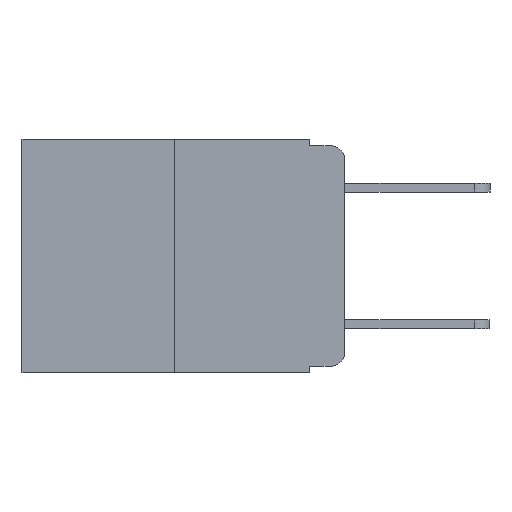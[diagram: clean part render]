
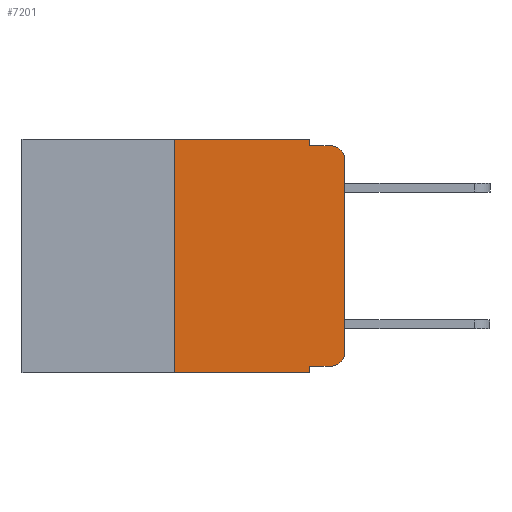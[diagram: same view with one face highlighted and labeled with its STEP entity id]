
A CAD part, left-side view. The second image highlights one B-rep face of the part: STEP entity #7201.
In plain terms, the highlighted planar face has unit normal (-1, 0, 0).
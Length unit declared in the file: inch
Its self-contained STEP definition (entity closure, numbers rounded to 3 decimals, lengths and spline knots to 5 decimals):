
#104 = VERTEX_POINT ( 'NONE', #10284 ) ;
#169 = CARTESIAN_POINT ( 'NONE',  ( 0., 0.051, 0. ) ) ;
#177 = VERTEX_POINT ( 'NONE', #1009 ) ;
#323 = VERTEX_POINT ( 'NONE', #8674 ) ;
#616 = VERTEX_POINT ( 'NONE', #6913 ) ;
#637 = ORIENTED_EDGE ( 'NONE', *, *, #11054, .F. ) ;
#781 = VECTOR ( 'NONE', #5788, 39.37008 ) ;
#1009 = CARTESIAN_POINT ( 'NONE',  ( 0., 0.02, -0.333 ) ) ;
#1039 = VERTEX_POINT ( 'NONE', #5582 ) ;
#1251 = ORIENTED_EDGE ( 'NONE', *, *, #3674, .T. ) ;
#1295 = VERTEX_POINT ( 'NONE', #3208 ) ;
#1386 = DIRECTION ( 'NONE',  ( -1., 0., 0. ) ) ;
#1568 = DIRECTION ( 'NONE',  ( 0., 0., -1. ) ) ;
#1674 = VECTOR ( 'NONE', #9213, 39.37008 ) ;
#1779 = VECTOR ( 'NONE', #10039, 39.37008 ) ;
#1827 = CARTESIAN_POINT ( 'NONE',  ( 0., 0.473, -0.343 ) ) ;
#2004 = LINE ( 'NONE', #1827, #8441 ) ;
#2006 = VERTEX_POINT ( 'NONE', #4079 ) ;
#2091 = ORIENTED_EDGE ( 'NONE', *, *, #7746, .F. ) ;
#2125 = EDGE_CURVE ( 'NONE', #323, #6568, #8767, .T. ) ;
#2162 = DIRECTION ( 'NONE',  ( -1., 0., 0. ) ) ;
#2323 = ORIENTED_EDGE ( 'NONE', *, *, #6759, .F. ) ;
#2906 = LINE ( 'NONE', #7291, #7264 ) ;
#3208 = CARTESIAN_POINT ( 'NONE',  ( 0., 0.25, 0. ) ) ;
#3257 = CIRCLE ( 'NONE', #7239, 0.02 ) ;
#3265 = CARTESIAN_POINT ( 'NONE',  ( 0., 0.051, -0.01 ) ) ;
#3390 = CARTESIAN_POINT ( 'NONE',  ( 0., 0.051, 0. ) ) ;
#3674 = EDGE_CURVE ( 'NONE', #177, #323, #3257, .T. ) ;
#3682 = ORIENTED_EDGE ( 'NONE', *, *, #8267, .F. ) ;
#3972 = VERTEX_POINT ( 'NONE', #10206 ) ;
#4079 = CARTESIAN_POINT ( 'NONE',  ( 0., 0.051, -0.01 ) ) ;
#4178 = PLANE ( 'NONE',  #7007 ) ;
#4637 = LINE ( 'NONE', #9237, #6681 ) ;
#4669 = VECTOR ( 'NONE', #5437, 39.37008 ) ;
#4691 = ORIENTED_EDGE ( 'NONE', *, *, #11189, .F. ) ;
#4791 = VERTEX_POINT ( 'NONE', #3390 ) ;
#4934 = LINE ( 'NONE', #11251, #4669 ) ;
#5046 = DIRECTION ( 'NONE',  ( 1., 0., 0. ) ) ;
#5053 = AXIS2_PLACEMENT_3D ( 'NONE', #6808, #1386, #7648 ) ;
#5229 = FACE_OUTER_BOUND ( 'NONE', #6292, .T. ) ;
#5437 = DIRECTION ( 'NONE',  ( 0., 0., 1. ) ) ;
#5490 = ORIENTED_EDGE ( 'NONE', *, *, #2125, .T. ) ;
#5582 = CARTESIAN_POINT ( 'NONE',  ( 0., 0.051, -0.343 ) ) ;
#5788 = DIRECTION ( 'NONE',  ( 0., 0., -1. ) ) ;
#5792 = ORIENTED_EDGE ( 'NONE', *, *, #6597, .T. ) ;
#5906 = DIRECTION ( 'NONE',  ( 0., -1., 0. ) ) ;
#5909 = EDGE_CURVE ( 'NONE', #104, #1039, #2004, .T. ) ;
#6289 = DIRECTION ( 'NONE',  ( 0., -1., 0. ) ) ;
#6292 = EDGE_LOOP ( 'NONE', ( #5490, #8907, #2323, #3682, #637, #2091, #10070, #4691, #5792, #1251 ) ) ;
#6568 = VERTEX_POINT ( 'NONE', #8056 ) ;
#6597 = EDGE_CURVE ( 'NONE', #616, #177, #2906, .T. ) ;
#6681 = VECTOR ( 'NONE', #5906, 39.37008 ) ;
#6759 = EDGE_CURVE ( 'NONE', #2006, #3972, #7658, .T. ) ;
#6808 = CARTESIAN_POINT ( 'NONE',  ( 0., 0.02, -0.03 ) ) ;
#6913 = CARTESIAN_POINT ( 'NONE',  ( 0., 0.051, -0.333 ) ) ;
#7007 = AXIS2_PLACEMENT_3D ( 'NONE', #10021, #5046, #10898 ) ;
#7201 = ADVANCED_FACE ( 'NONE', ( #5229 ), #4178, .F. ) ;
#7239 = AXIS2_PLACEMENT_3D ( 'NONE', #7456, #2162, #8277 ) ;
#7264 = VECTOR ( 'NONE', #11318, 39.37008 ) ;
#7291 = CARTESIAN_POINT ( 'NONE',  ( 0., 0.051, -0.333 ) ) ;
#7456 = CARTESIAN_POINT ( 'NONE',  ( 0., 0.02, -0.313 ) ) ;
#7613 = VECTOR ( 'NONE', #1568, 39.37008 ) ;
#7648 = DIRECTION ( 'NONE',  ( 0., 0., -1. ) ) ;
#7658 = LINE ( 'NONE', #3265, #1674 ) ;
#7746 = EDGE_CURVE ( 'NONE', #104, #1295, #4934, .T. ) ;
#7881 = LINE ( 'NONE', #8578, #7613 ) ;
#8056 = CARTESIAN_POINT ( 'NONE',  ( 0., 0., -0.03 ) ) ;
#8267 = EDGE_CURVE ( 'NONE', #4791, #2006, #9845, .T. ) ;
#8277 = DIRECTION ( 'NONE',  ( 0., 0., -1. ) ) ;
#8441 = VECTOR ( 'NONE', #6289, 39.37008 ) ;
#8578 = CARTESIAN_POINT ( 'NONE',  ( 0., 0.051, 0. ) ) ;
#8674 = CARTESIAN_POINT ( 'NONE',  ( 0., 0., -0.313 ) ) ;
#8767 = LINE ( 'NONE', #10879, #1779 ) ;
#8907 = ORIENTED_EDGE ( 'NONE', *, *, #11010, .T. ) ;
#9213 = DIRECTION ( 'NONE',  ( 0., -1., 0. ) ) ;
#9237 = CARTESIAN_POINT ( 'NONE',  ( 0., 0.473, 0. ) ) ;
#9845 = LINE ( 'NONE', #169, #781 ) ;
#10021 = CARTESIAN_POINT ( 'NONE',  ( 0., 0.473, 0. ) ) ;
#10039 = DIRECTION ( 'NONE',  ( 0., 0., 1. ) ) ;
#10070 = ORIENTED_EDGE ( 'NONE', *, *, #5909, .T. ) ;
#10206 = CARTESIAN_POINT ( 'NONE',  ( 0., 0.02, -0.01 ) ) ;
#10284 = CARTESIAN_POINT ( 'NONE',  ( 0., 0.25, -0.343 ) ) ;
#10879 = CARTESIAN_POINT ( 'NONE',  ( 0., 0., 0. ) ) ;
#10898 = DIRECTION ( 'NONE',  ( 0., 0., -1. ) ) ;
#11010 = EDGE_CURVE ( 'NONE', #6568, #3972, #11265, .T. ) ;
#11054 = EDGE_CURVE ( 'NONE', #1295, #4791, #4637, .T. ) ;
#11189 = EDGE_CURVE ( 'NONE', #616, #1039, #7881, .T. ) ;
#11251 = CARTESIAN_POINT ( 'NONE',  ( 0., 0.25, 0. ) ) ;
#11265 = CIRCLE ( 'NONE', #5053, 0.02 ) ;
#11318 = DIRECTION ( 'NONE',  ( 0., -1., 0. ) ) ;
